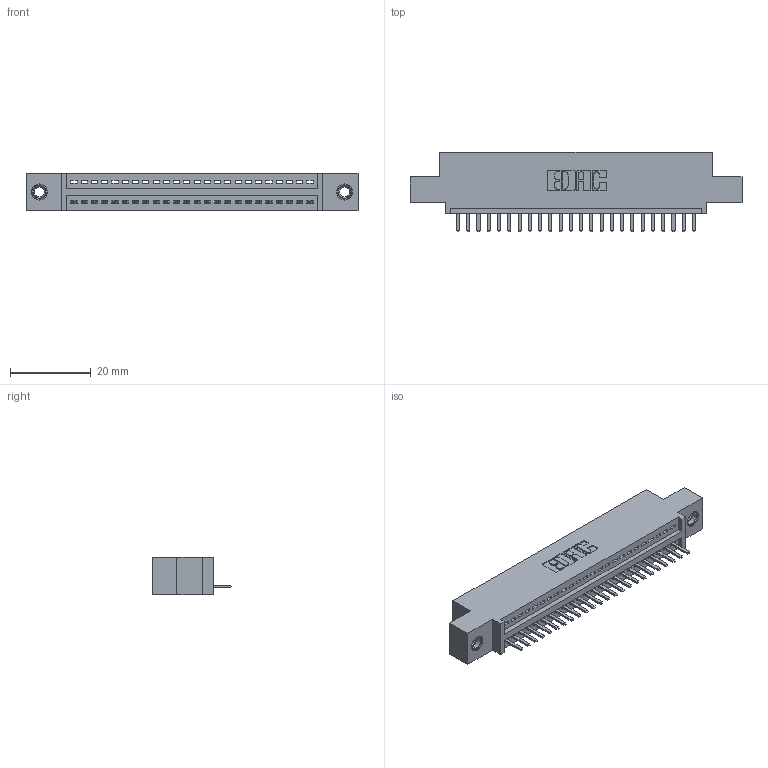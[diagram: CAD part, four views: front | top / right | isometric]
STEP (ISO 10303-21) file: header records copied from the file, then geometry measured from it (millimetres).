
FILE_DESCRIPTION (( 'STEP AP203' ), '1' );
FILE_NAME ('395-024-520-407.STEP', '2018-11-08T14:43:55', ( '' ), ( '' ), 'SwSTEP 2.0', 'SolidWorks 2016', '' );
FILE_SCHEMA (( 'CONFIG_CONTROL_DESIGN' ));
Length unit declared in the file: inch
Products named in the file (4): 345-250-001_345-250-005-103; 345 Part_0.110 Offset - 0.156 Dia-TI; 345-292-001_345-293-120; 395-024-520-407
Assembly tree (27 placements, depth 2):
  395-024-520-407
    345 Part_0.110 Offset - 0.156 Dia-TI
    345-292-001_345-293-120  x24
    345-250-001_345-250-005-103  x2
Bounding box: 82.17 x 19.68 x 9.4 mm (x, y, z)
Volume: 7501.1 mm3; surface area: 9612.3 mm2
Topology: 27 solids, 27 shells, 1678 faces, 4905 edges, 3198 vertices
Faces by surface type: plane 1124, cylinder 538, cone 12, torus 4
Entity records: 21918 total; most frequent: CARTESIAN_POINT 3791, ORIENTED_EDGE 3730, DIRECTION 3351, EDGE_CURVE 1865, VECTOR 1613, LINE 1613, VERTEX_POINT 1236, AXIS2_PLACEMENT_3D 869
